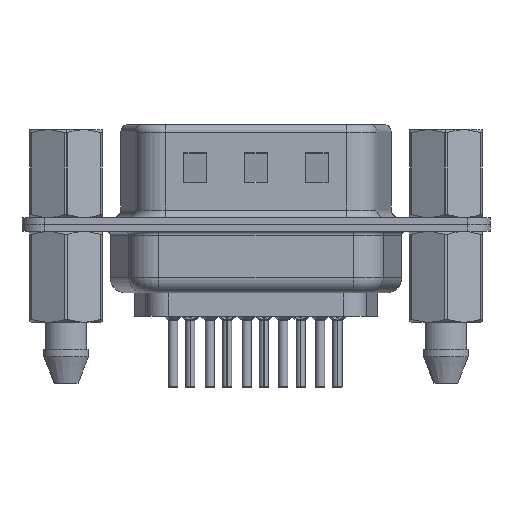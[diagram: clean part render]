
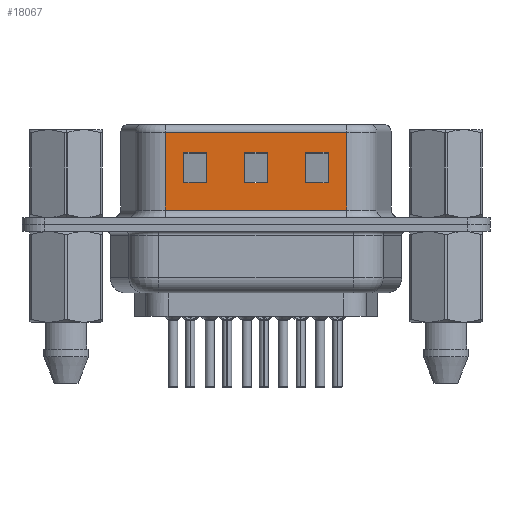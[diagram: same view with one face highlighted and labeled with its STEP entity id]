
A CAD part, front view. The second image highlights one B-rep face of the part: STEP entity #18067.
In plain terms, the highlighted planar face has unit normal (0, -1, 0).
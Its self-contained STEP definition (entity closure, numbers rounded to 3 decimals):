
#233 = VECTOR ( 'NONE', #5331, 1000. ) ;
#350 = CARTESIAN_POINT ( 'NONE',  ( 17.245, -4.64, 2.755 ) ) ;
#722 = DIRECTION ( 'NONE',  ( 0., 0., 1. ) ) ;
#756 = CARTESIAN_POINT ( 'NONE',  ( 7.745, -4.64, 6.57 ) ) ;
#806 = CARTESIAN_POINT ( 'NONE',  ( 18.474, -4.64, 2.755 ) ) ;
#870 = EDGE_CURVE ( 'NONE', #2465, #5036, #23922, .T. ) ;
#874 = VERTEX_POINT ( 'NONE', #24042 ) ;
#1335 = CARTESIAN_POINT ( 'NONE',  ( 6.516, -4.64, 0.95 ) ) ;
#1355 = CARTESIAN_POINT ( 'NONE',  ( 18.474, -4.64, 0.95 ) ) ;
#1809 = CARTESIAN_POINT ( 'NONE',  ( 14.474, -4.64, 2.755 ) ) ;
#1850 = CARTESIAN_POINT ( 'NONE',  ( 11.745, -4.64, 6.57 ) ) ;
#2308 = VECTOR ( 'NONE', #22222, 1000. ) ;
#2465 = VERTEX_POINT ( 'NONE', #26173 ) ;
#2498 = CARTESIAN_POINT ( 'NONE',  ( 9.245, -4.64, 2.755 ) ) ;
#2541 = CARTESIAN_POINT ( 'NONE',  ( 18.474, -4.64, 4.755 ) ) ;
#2923 = CARTESIAN_POINT ( 'NONE',  ( 22.474, -4.64, 4.755 ) ) ;
#2994 = CARTESIAN_POINT ( 'NONE',  ( 13.245, -4.64, 2.755 ) ) ;
#3237 = EDGE_CURVE ( 'NONE', #8485, #17893, #5265, .T. ) ;
#3268 = CARTESIAN_POINT ( 'NONE',  ( 18.474, -4.64, 6.57 ) ) ;
#3425 = EDGE_CURVE ( 'NONE', #16236, #8394, #7030, .T. ) ;
#3897 = VERTEX_POINT ( 'NONE', #20645 ) ;
#3967 = EDGE_CURVE ( 'NONE', #19206, #21180, #7002, .T. ) ;
#4347 = VECTOR ( 'NONE', #4847, 1000. ) ;
#4847 = DIRECTION ( 'NONE',  ( 1., 0., 0. ) ) ;
#5036 = VERTEX_POINT ( 'NONE', #12055 ) ;
#5229 = DIRECTION ( 'NONE',  ( 1., 0., 0. ) ) ;
#5265 = LINE ( 'NONE', #19732, #16570 ) ;
#5331 = DIRECTION ( 'NONE',  ( 1., 0., 0. ) ) ;
#5507 = CARTESIAN_POINT ( 'NONE',  ( 17.245, -4.64, 4.755 ) ) ;
#5661 = EDGE_CURVE ( 'NONE', #8485, #24727, #26371, .T. ) ;
#5740 = PLANE ( 'NONE',  #22594 ) ;
#5889 = ORIENTED_EDGE ( 'NONE', *, *, #16888, .T. ) ;
#6165 = DIRECTION ( 'NONE',  ( -1., 0., 0. ) ) ;
#6913 = ORIENTED_EDGE ( 'NONE', *, *, #10488, .T. ) ;
#6986 = ORIENTED_EDGE ( 'NONE', *, *, #16189, .T. ) ;
#7002 = LINE ( 'NONE', #806, #11605 ) ;
#7030 = LINE ( 'NONE', #20527, #25076 ) ;
#7216 = VECTOR ( 'NONE', #25970, 1000. ) ;
#7619 = FACE_BOUND ( 'NONE', #13462, .T. ) ;
#8034 = DIRECTION ( 'NONE',  ( 0., 1., 0. ) ) ;
#8170 = LINE ( 'NONE', #22561, #26206 ) ;
#8340 = VECTOR ( 'NONE', #14575, 1000. ) ;
#8352 = FACE_BOUND ( 'NONE', #13410, .T. ) ;
#8394 = VERTEX_POINT ( 'NONE', #350 ) ;
#8485 = VERTEX_POINT ( 'NONE', #16596 ) ;
#8651 = VERTEX_POINT ( 'NONE', #1335 ) ;
#9043 = DIRECTION ( 'NONE',  ( -1., 0., 0. ) ) ;
#9222 = CARTESIAN_POINT ( 'NONE',  ( 15.745, -4.64, 6.57 ) ) ;
#9594 = ORIENTED_EDGE ( 'NONE', *, *, #3967, .T. ) ;
#9726 = EDGE_CURVE ( 'NONE', #8394, #3897, #14036, .T. ) ;
#9798 = DIRECTION ( 'NONE',  ( 1., 0., 0. ) ) ;
#10488 = EDGE_CURVE ( 'NONE', #23602, #16236, #11172, .T. ) ;
#10877 = ORIENTED_EDGE ( 'NONE', *, *, #3237, .T. ) ;
#10882 = VECTOR ( 'NONE', #19137, 1000. ) ;
#11172 = LINE ( 'NONE', #2923, #28472 ) ;
#11478 = DIRECTION ( 'NONE',  ( 0., 0., 1. ) ) ;
#11509 = ORIENTED_EDGE ( 'NONE', *, *, #3425, .T. ) ;
#11605 = VECTOR ( 'NONE', #27944, 1000. ) ;
#11767 = EDGE_CURVE ( 'NONE', #21180, #23139, #15348, .T. ) ;
#11903 = VECTOR ( 'NONE', #722, 1000. ) ;
#12055 = CARTESIAN_POINT ( 'NONE',  ( 7.745, -4.64, 4.755 ) ) ;
#12244 = CARTESIAN_POINT ( 'NONE',  ( 11.745, -4.64, 2.755 ) ) ;
#12309 = CARTESIAN_POINT ( 'NONE',  ( 6.516, -4.64, 6.57 ) ) ;
#12959 = FACE_BOUND ( 'NONE', #18787, .T. ) ;
#13410 = EDGE_LOOP ( 'NONE', ( #11509, #13433, #19725, #6913 ) ) ;
#13433 = ORIENTED_EDGE ( 'NONE', *, *, #9726, .T. ) ;
#13462 = EDGE_LOOP ( 'NONE', ( #24835, #23270, #9594, #20144 ) ) ;
#13682 = CARTESIAN_POINT ( 'NONE',  ( 22.474, -4.64, 2.755 ) ) ;
#14036 = LINE ( 'NONE', #13682, #25338 ) ;
#14330 = CARTESIAN_POINT ( 'NONE',  ( 14.474, -4.64, 4.755 ) ) ;
#14575 = DIRECTION ( 'NONE',  ( 0., 0., -1. ) ) ;
#14602 = CARTESIAN_POINT ( 'NONE',  ( 13.245, -4.64, 6.57 ) ) ;
#15348 = LINE ( 'NONE', #1850, #25688 ) ;
#15849 = CARTESIAN_POINT ( 'NONE',  ( 6.516, -4.64, 6.07 ) ) ;
#15937 = LINE ( 'NONE', #18798, #27946 ) ;
#15992 = LINE ( 'NONE', #9222, #26608 ) ;
#15993 = EDGE_CURVE ( 'NONE', #3897, #23602, #15992, .T. ) ;
#16189 = EDGE_CURVE ( 'NONE', #5036, #27511, #25058, .T. ) ;
#16236 = VERTEX_POINT ( 'NONE', #5507 ) ;
#16570 = VECTOR ( 'NONE', #6165, 1000. ) ;
#16596 = CARTESIAN_POINT ( 'NONE',  ( 18.474, -4.64, 6.07 ) ) ;
#16687 = VERTEX_POINT ( 'NONE', #2498 ) ;
#16888 = EDGE_CURVE ( 'NONE', #17893, #8651, #22896, .T. ) ;
#17714 = DIRECTION ( 'NONE',  ( 0., 0., 1. ) ) ;
#17893 = VERTEX_POINT ( 'NONE', #15849 ) ;
#18067 = ADVANCED_FACE ( 'NONE', ( #12959, #8352, #7619, #18959 ), #5740, .F. ) ;
#18537 = LINE ( 'NONE', #14602, #7216 ) ;
#18787 = EDGE_LOOP ( 'NONE', ( #27149, #25114, #27005, #6986 ) ) ;
#18798 = CARTESIAN_POINT ( 'NONE',  ( 18.474, -4.64, 0.95 ) ) ;
#18959 = FACE_OUTER_BOUND ( 'NONE', #25629, .T. ) ;
#19137 = DIRECTION ( 'NONE',  ( 0., 0., -1. ) ) ;
#19206 = VERTEX_POINT ( 'NONE', #2994 ) ;
#19725 = ORIENTED_EDGE ( 'NONE', *, *, #15993, .T. ) ;
#19732 = CARTESIAN_POINT ( 'NONE',  ( 18.474, -4.64, 6.07 ) ) ;
#19802 = EDGE_CURVE ( 'NONE', #23139, #874, #28402, .T. ) ;
#20144 = ORIENTED_EDGE ( 'NONE', *, *, #11767, .T. ) ;
#20527 = CARTESIAN_POINT ( 'NONE',  ( 17.245, -4.64, 6.57 ) ) ;
#20645 = CARTESIAN_POINT ( 'NONE',  ( 15.745, -4.64, 2.755 ) ) ;
#20904 = CARTESIAN_POINT ( 'NONE',  ( 15.745, -4.64, 4.755 ) ) ;
#21180 = VERTEX_POINT ( 'NONE', #12244 ) ;
#22222 = DIRECTION ( 'NONE',  ( -1., 0., 0. ) ) ;
#22288 = EDGE_CURVE ( 'NONE', #27511, #16687, #8170, .T. ) ;
#22505 = EDGE_CURVE ( 'NONE', #8651, #24727, #15937, .T. ) ;
#22561 = CARTESIAN_POINT ( 'NONE',  ( 9.245, -4.64, 6.57 ) ) ;
#22594 = AXIS2_PLACEMENT_3D ( 'NONE', #26026, #8034, #23832 ) ;
#22781 = DIRECTION ( 'NONE',  ( 0., 0., -1. ) ) ;
#22896 = LINE ( 'NONE', #12309, #10882 ) ;
#23139 = VERTEX_POINT ( 'NONE', #25471 ) ;
#23270 = ORIENTED_EDGE ( 'NONE', *, *, #27058, .T. ) ;
#23602 = VERTEX_POINT ( 'NONE', #20904 ) ;
#23832 = DIRECTION ( 'NONE',  ( 0., 0., 1. ) ) ;
#23922 = LINE ( 'NONE', #756, #11903 ) ;
#24042 = CARTESIAN_POINT ( 'NONE',  ( 13.245, -4.64, 4.755 ) ) ;
#24146 = ORIENTED_EDGE ( 'NONE', *, *, #5661, .F. ) ;
#24727 = VERTEX_POINT ( 'NONE', #1355 ) ;
#24835 = ORIENTED_EDGE ( 'NONE', *, *, #19802, .T. ) ;
#25058 = LINE ( 'NONE', #14330, #233 ) ;
#25076 = VECTOR ( 'NONE', #22781, 1000. ) ;
#25114 = ORIENTED_EDGE ( 'NONE', *, *, #25522, .T. ) ;
#25338 = VECTOR ( 'NONE', #9043, 1000. ) ;
#25471 = CARTESIAN_POINT ( 'NONE',  ( 11.745, -4.64, 4.755 ) ) ;
#25522 = EDGE_CURVE ( 'NONE', #16687, #2465, #27113, .T. ) ;
#25629 = EDGE_LOOP ( 'NONE', ( #24146, #10877, #5889, #28748 ) ) ;
#25688 = VECTOR ( 'NONE', #17714, 1000. ) ;
#25755 = CARTESIAN_POINT ( 'NONE',  ( 9.245, -4.64, 4.755 ) ) ;
#25970 = DIRECTION ( 'NONE',  ( 0., 0., -1. ) ) ;
#26026 = CARTESIAN_POINT ( 'NONE',  ( 18.474, -4.64, 6.57 ) ) ;
#26173 = CARTESIAN_POINT ( 'NONE',  ( 7.745, -4.64, 2.755 ) ) ;
#26206 = VECTOR ( 'NONE', #29246, 1000. ) ;
#26371 = LINE ( 'NONE', #3268, #8340 ) ;
#26608 = VECTOR ( 'NONE', #11478, 1000. ) ;
#27005 = ORIENTED_EDGE ( 'NONE', *, *, #870, .T. ) ;
#27058 = EDGE_CURVE ( 'NONE', #874, #19206, #18537, .T. ) ;
#27113 = LINE ( 'NONE', #1809, #2308 ) ;
#27149 = ORIENTED_EDGE ( 'NONE', *, *, #22288, .T. ) ;
#27511 = VERTEX_POINT ( 'NONE', #25755 ) ;
#27944 = DIRECTION ( 'NONE',  ( -1., 0., 0. ) ) ;
#27946 = VECTOR ( 'NONE', #9798, 1000. ) ;
#28402 = LINE ( 'NONE', #2541, #4347 ) ;
#28472 = VECTOR ( 'NONE', #5229, 1000. ) ;
#28748 = ORIENTED_EDGE ( 'NONE', *, *, #22505, .T. ) ;
#29246 = DIRECTION ( 'NONE',  ( 0., 0., -1. ) ) ;
